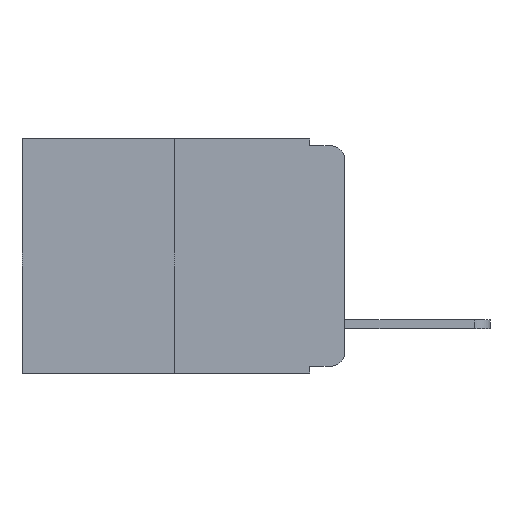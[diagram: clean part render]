
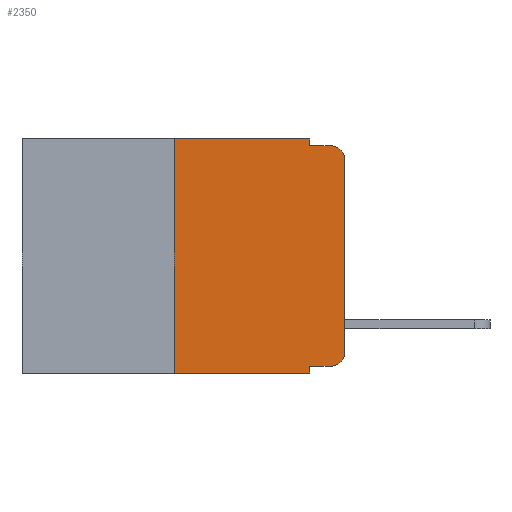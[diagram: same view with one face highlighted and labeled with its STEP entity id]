
A CAD part, left-side view. The second image highlights one B-rep face of the part: STEP entity #2350.
In plain terms, the highlighted planar face has unit normal (-1, 0, 0).
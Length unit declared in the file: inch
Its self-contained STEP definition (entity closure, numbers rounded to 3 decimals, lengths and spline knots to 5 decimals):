
#167 = DIRECTION ( 'NONE',  ( 0., 0., 1. ) ) ;
#192 = DIRECTION ( 'NONE',  ( 0., 0., -1. ) ) ;
#348 = CARTESIAN_POINT ( 'NONE',  ( 0., 0.473, -0.343 ) ) ;
#353 = VECTOR ( 'NONE', #9630, 39.37008 ) ;
#418 = CARTESIAN_POINT ( 'NONE',  ( 0., 0.25, 0. ) ) ;
#478 = CARTESIAN_POINT ( 'NONE',  ( 0., 0.051, 0. ) ) ;
#487 = EDGE_CURVE ( 'NONE', #6174, #1006, #6788, .T. ) ;
#585 = EDGE_CURVE ( 'NONE', #2087, #1750, #10753, .T. ) ;
#790 = EDGE_CURVE ( 'NONE', #2087, #9795, #7733, .T. ) ;
#885 = LINE ( 'NONE', #348, #5437 ) ;
#913 = EDGE_CURVE ( 'NONE', #9795, #4196, #4463, .T. ) ;
#1006 = VERTEX_POINT ( 'NONE', #418 ) ;
#1200 = VECTOR ( 'NONE', #7034, 39.37008 ) ;
#1315 = CARTESIAN_POINT ( 'NONE',  ( 0., 0., -0.03 ) ) ;
#1337 = DIRECTION ( 'NONE',  ( 0., -1., 0. ) ) ;
#1359 = CARTESIAN_POINT ( 'NONE',  ( 0., 0.051, -0.01 ) ) ;
#1750 = VERTEX_POINT ( 'NONE', #8866 ) ;
#1873 = VERTEX_POINT ( 'NONE', #2615 ) ;
#2087 = VERTEX_POINT ( 'NONE', #8344 ) ;
#2138 = CARTESIAN_POINT ( 'NONE',  ( 0., 0.051, 0. ) ) ;
#2156 = DIRECTION ( 'NONE',  ( -1., 0., 0. ) ) ;
#2350 = ADVANCED_FACE ( 'NONE', ( #7009 ), #4801, .F. ) ;
#2533 = DIRECTION ( 'NONE',  ( 0., 0., -1. ) ) ;
#2615 = CARTESIAN_POINT ( 'NONE',  ( 0., 0.051, 0. ) ) ;
#2747 = CARTESIAN_POINT ( 'NONE',  ( 0., 0.25, 0. ) ) ;
#2762 = DIRECTION ( 'NONE',  ( 0., 0., 1. ) ) ;
#2880 = LINE ( 'NONE', #1359, #5279 ) ;
#2972 = CARTESIAN_POINT ( 'NONE',  ( 0., 0.051, -0.01 ) ) ;
#3137 = CARTESIAN_POINT ( 'NONE',  ( 0., 0.02, -0.333 ) ) ;
#3538 = EDGE_LOOP ( 'NONE', ( #8747, #10808, #5230, #5254, #5527, #10499, #7598, #6437, #8661, #6899 ) ) ;
#3665 = LINE ( 'NONE', #5132, #1200 ) ;
#4196 = VERTEX_POINT ( 'NONE', #6753 ) ;
#4459 = LINE ( 'NONE', #478, #8298 ) ;
#4463 = CIRCLE ( 'NONE', #6905, 0.02 ) ;
#4801 = PLANE ( 'NONE',  #8674 ) ;
#5132 = CARTESIAN_POINT ( 'NONE',  ( 0., 0.473, 0. ) ) ;
#5230 = ORIENTED_EDGE ( 'NONE', *, *, #10621, .F. ) ;
#5254 = ORIENTED_EDGE ( 'NONE', *, *, #10690, .F. ) ;
#5279 = VECTOR ( 'NONE', #7296, 39.37008 ) ;
#5437 = VECTOR ( 'NONE', #1337, 39.37008 ) ;
#5527 = ORIENTED_EDGE ( 'NONE', *, *, #8462, .F. ) ;
#6002 = VECTOR ( 'NONE', #167, 39.37008 ) ;
#6174 = VERTEX_POINT ( 'NONE', #10708 ) ;
#6437 = ORIENTED_EDGE ( 'NONE', *, *, #585, .F. ) ;
#6556 = VECTOR ( 'NONE', #2762, 39.37008 ) ;
#6753 = CARTESIAN_POINT ( 'NONE',  ( 0., 0., -0.313 ) ) ;
#6788 = LINE ( 'NONE', #2747, #6556 ) ;
#6899 = ORIENTED_EDGE ( 'NONE', *, *, #913, .T. ) ;
#6905 = AXIS2_PLACEMENT_3D ( 'NONE', #10261, #7661, #7430 ) ;
#6915 = VECTOR ( 'NONE', #192, 39.37008 ) ;
#7009 = FACE_OUTER_BOUND ( 'NONE', #3538, .T. ) ;
#7034 = DIRECTION ( 'NONE',  ( 0., -1., 0. ) ) ;
#7199 = CARTESIAN_POINT ( 'NONE',  ( 0., 0.02, -0.03 ) ) ;
#7209 = VERTEX_POINT ( 'NONE', #2972 ) ;
#7296 = DIRECTION ( 'NONE',  ( 0., -1., 0. ) ) ;
#7376 = VERTEX_POINT ( 'NONE', #9503 ) ;
#7430 = DIRECTION ( 'NONE',  ( 0., 0., -1. ) ) ;
#7598 = ORIENTED_EDGE ( 'NONE', *, *, #9832, .T. ) ;
#7661 = DIRECTION ( 'NONE',  ( -1., 0., 0. ) ) ;
#7733 = LINE ( 'NONE', #9544, #353 ) ;
#7947 = DIRECTION ( 'NONE',  ( 0., 0., -1. ) ) ;
#8298 = VECTOR ( 'NONE', #2533, 39.37008 ) ;
#8344 = CARTESIAN_POINT ( 'NONE',  ( 0., 0.051, -0.333 ) ) ;
#8462 = EDGE_CURVE ( 'NONE', #1006, #1873, #3665, .T. ) ;
#8661 = ORIENTED_EDGE ( 'NONE', *, *, #790, .T. ) ;
#8674 = AXIS2_PLACEMENT_3D ( 'NONE', #9569, #10271, #9536 ) ;
#8747 = ORIENTED_EDGE ( 'NONE', *, *, #10502, .T. ) ;
#8855 = AXIS2_PLACEMENT_3D ( 'NONE', #7199, #2156, #7947 ) ;
#8866 = CARTESIAN_POINT ( 'NONE',  ( 0., 0.051, -0.343 ) ) ;
#9133 = VERTEX_POINT ( 'NONE', #1315 ) ;
#9408 = CARTESIAN_POINT ( 'NONE',  ( 0., 0., 0. ) ) ;
#9503 = CARTESIAN_POINT ( 'NONE',  ( 0., 0.02, -0.01 ) ) ;
#9536 = DIRECTION ( 'NONE',  ( 0., 0., -1. ) ) ;
#9544 = CARTESIAN_POINT ( 'NONE',  ( 0., 0.051, -0.333 ) ) ;
#9569 = CARTESIAN_POINT ( 'NONE',  ( 0., 0.473, 0. ) ) ;
#9630 = DIRECTION ( 'NONE',  ( 0., -1., 0. ) ) ;
#9795 = VERTEX_POINT ( 'NONE', #3137 ) ;
#9803 = CIRCLE ( 'NONE', #8855, 0.02 ) ;
#9832 = EDGE_CURVE ( 'NONE', #6174, #1750, #885, .T. ) ;
#10055 = LINE ( 'NONE', #9408, #6002 ) ;
#10261 = CARTESIAN_POINT ( 'NONE',  ( 0., 0.02, -0.313 ) ) ;
#10271 = DIRECTION ( 'NONE',  ( 1., 0., 0. ) ) ;
#10499 = ORIENTED_EDGE ( 'NONE', *, *, #487, .F. ) ;
#10502 = EDGE_CURVE ( 'NONE', #4196, #9133, #10055, .T. ) ;
#10534 = EDGE_CURVE ( 'NONE', #9133, #7376, #9803, .T. ) ;
#10621 = EDGE_CURVE ( 'NONE', #7209, #7376, #2880, .T. ) ;
#10690 = EDGE_CURVE ( 'NONE', #1873, #7209, #4459, .T. ) ;
#10708 = CARTESIAN_POINT ( 'NONE',  ( 0., 0.25, -0.343 ) ) ;
#10753 = LINE ( 'NONE', #2138, #6915 ) ;
#10808 = ORIENTED_EDGE ( 'NONE', *, *, #10534, .T. ) ;
